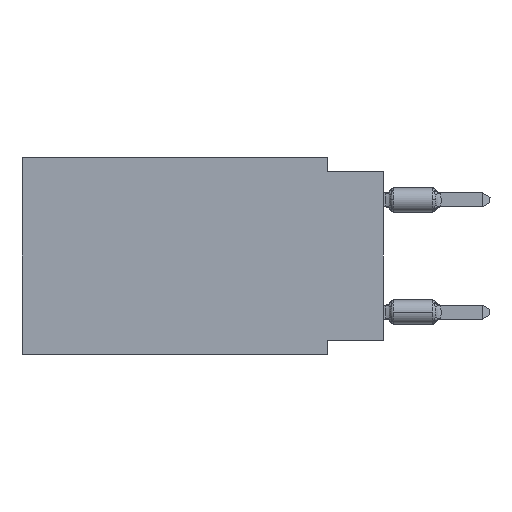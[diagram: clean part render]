
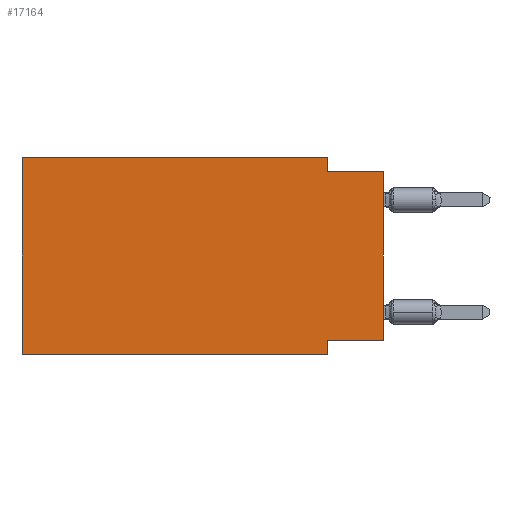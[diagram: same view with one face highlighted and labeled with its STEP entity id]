
A CAD part, left-side view. The second image highlights one B-rep face of the part: STEP entity #17164.
In plain terms, the highlighted planar face has unit normal (-1, 0, 0).
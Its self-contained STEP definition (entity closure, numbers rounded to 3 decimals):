
#393 = CARTESIAN_POINT ( 'NONE',  ( 0., 2.54, -8.255 ) ) ;
#741 = VERTEX_POINT ( 'NONE', #14095 ) ;
#905 = LINE ( 'NONE', #10170, #8812 ) ;
#958 = CARTESIAN_POINT ( 'NONE',  ( 0., 0., 0. ) ) ;
#1184 = FACE_OUTER_BOUND ( 'NONE', #8278, .T. ) ;
#1526 = VECTOR ( 'NONE', #27014, 1000. ) ;
#1857 = CARTESIAN_POINT ( 'NONE',  ( 0., 16.383, 0. ) ) ;
#1996 = LINE ( 'NONE', #1857, #10190 ) ;
#2284 = EDGE_CURVE ( 'NONE', #17820, #25648, #2809, .T. ) ;
#2809 = LINE ( 'NONE', #12375, #8031 ) ;
#3264 = VECTOR ( 'NONE', #19668, 1000. ) ;
#4077 = EDGE_CURVE ( 'NONE', #741, #17820, #16903, .T. ) ;
#4388 = CARTESIAN_POINT ( 'NONE',  ( 0., 2.54, -0.635 ) ) ;
#4497 = CARTESIAN_POINT ( 'NONE',  ( 0., 2.54, -8.89 ) ) ;
#4679 = CARTESIAN_POINT ( 'NONE',  ( 0., 16.383, -8.89 ) ) ;
#5337 = ORIENTED_EDGE ( 'NONE', *, *, #29095, .T. ) ;
#6127 = ORIENTED_EDGE ( 'NONE', *, *, #7585, .F. ) ;
#6546 = AXIS2_PLACEMENT_3D ( 'NONE', #12607, #22305, #27093 ) ;
#7585 = EDGE_CURVE ( 'NONE', #22291, #741, #1996, .T. ) ;
#7669 = CARTESIAN_POINT ( 'NONE',  ( 0., 2.54, 0. ) ) ;
#8031 = VECTOR ( 'NONE', #23769, 1000. ) ;
#8278 = EDGE_LOOP ( 'NONE', ( #5337, #27386, #29563, #6127, #13484, #28385, #11849, #18425 ) ) ;
#8669 = CARTESIAN_POINT ( 'NONE',  ( 0., 2.54, -8.89 ) ) ;
#8812 = VECTOR ( 'NONE', #19561, 1000. ) ;
#9490 = DIRECTION ( 'NONE',  ( 0., 0., 1. ) ) ;
#9549 = EDGE_CURVE ( 'NONE', #26835, #22969, #905, .T. ) ;
#10170 = CARTESIAN_POINT ( 'NONE',  ( 0., 16.383, -8.89 ) ) ;
#10190 = VECTOR ( 'NONE', #20511, 1000. ) ;
#10578 = VERTEX_POINT ( 'NONE', #25603 ) ;
#11849 = ORIENTED_EDGE ( 'NONE', *, *, #20109, .F. ) ;
#12110 = LINE ( 'NONE', #16581, #3264 ) ;
#12375 = CARTESIAN_POINT ( 'NONE',  ( 0., 0., -0.635 ) ) ;
#12607 = CARTESIAN_POINT ( 'NONE',  ( 0., 16.383, 0. ) ) ;
#12890 = EDGE_CURVE ( 'NONE', #26835, #22291, #27839, .T. ) ;
#13052 = VERTEX_POINT ( 'NONE', #393 ) ;
#13484 = ORIENTED_EDGE ( 'NONE', *, *, #12890, .F. ) ;
#13891 = DIRECTION ( 'NONE',  ( 0., 0., -1. ) ) ;
#14095 = CARTESIAN_POINT ( 'NONE',  ( 0., 2.54, 0. ) ) ;
#15000 = LINE ( 'NONE', #958, #1526 ) ;
#15235 = PLANE ( 'NONE',  #6546 ) ;
#16581 = CARTESIAN_POINT ( 'NONE',  ( 0., 0., -8.255 ) ) ;
#16753 = CARTESIAN_POINT ( 'NONE',  ( 0., 16.383, 0. ) ) ;
#16903 = LINE ( 'NONE', #7669, #21395 ) ;
#17164 = ADVANCED_FACE ( 'NONE', ( #1184 ), #15235, .F. ) ;
#17318 = VECTOR ( 'NONE', #9490, 1000. ) ;
#17820 = VERTEX_POINT ( 'NONE', #4388 ) ;
#18425 = ORIENTED_EDGE ( 'NONE', *, *, #26549, .F. ) ;
#19561 = DIRECTION ( 'NONE',  ( 0., -1., 0. ) ) ;
#19668 = DIRECTION ( 'NONE',  ( 0., 1., 0. ) ) ;
#20109 = EDGE_CURVE ( 'NONE', #13052, #22969, #27327, .T. ) ;
#20511 = DIRECTION ( 'NONE',  ( 0., -1., 0. ) ) ;
#21395 = VECTOR ( 'NONE', #24157, 1000. ) ;
#22291 = VERTEX_POINT ( 'NONE', #16753 ) ;
#22305 = DIRECTION ( 'NONE',  ( 1., 0., 0. ) ) ;
#22969 = VERTEX_POINT ( 'NONE', #8669 ) ;
#23278 = CARTESIAN_POINT ( 'NONE',  ( 0., 0., -0.635 ) ) ;
#23769 = DIRECTION ( 'NONE',  ( 0., -1., 0. ) ) ;
#24157 = DIRECTION ( 'NONE',  ( 0., 0., -1. ) ) ;
#25603 = CARTESIAN_POINT ( 'NONE',  ( 0., 0., -8.255 ) ) ;
#25648 = VERTEX_POINT ( 'NONE', #23278 ) ;
#26549 = EDGE_CURVE ( 'NONE', #10578, #13052, #12110, .T. ) ;
#26835 = VERTEX_POINT ( 'NONE', #4679 ) ;
#27014 = DIRECTION ( 'NONE',  ( 0., 0., 1. ) ) ;
#27093 = DIRECTION ( 'NONE',  ( 0., 0., -1. ) ) ;
#27327 = LINE ( 'NONE', #4497, #27415 ) ;
#27386 = ORIENTED_EDGE ( 'NONE', *, *, #2284, .F. ) ;
#27415 = VECTOR ( 'NONE', #13891, 1000. ) ;
#27839 = LINE ( 'NONE', #30308, #17318 ) ;
#28385 = ORIENTED_EDGE ( 'NONE', *, *, #9549, .T. ) ;
#29095 = EDGE_CURVE ( 'NONE', #10578, #25648, #15000, .T. ) ;
#29563 = ORIENTED_EDGE ( 'NONE', *, *, #4077, .F. ) ;
#30308 = CARTESIAN_POINT ( 'NONE',  ( 0., 16.383, 0. ) ) ;
